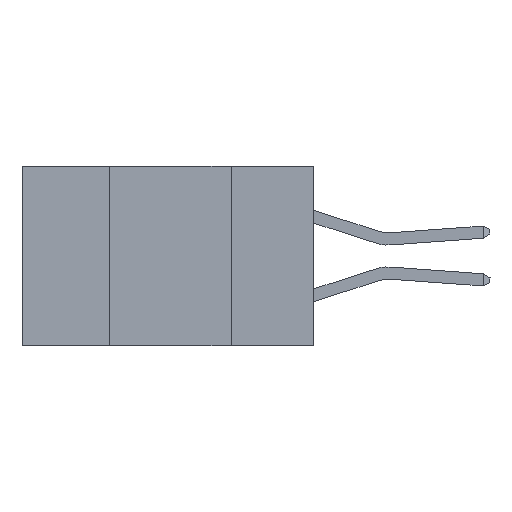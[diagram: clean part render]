
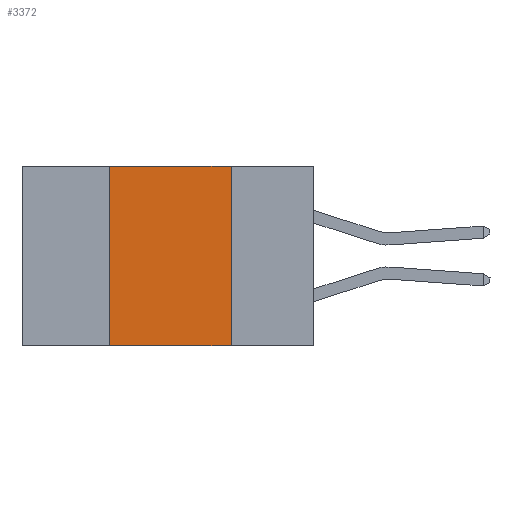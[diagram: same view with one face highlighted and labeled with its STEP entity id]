
A CAD part, left-side view. The second image highlights one B-rep face of the part: STEP entity #3372.
In plain terms, the highlighted planar face has unit normal (-1, 0, 0).
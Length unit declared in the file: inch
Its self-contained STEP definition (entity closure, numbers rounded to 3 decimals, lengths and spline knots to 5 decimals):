
#1549 = DIRECTION ( 'NONE',  ( 0., 0., -1. ) ) ;
#2661 = VECTOR ( 'NONE', #29546, 39.37008 ) ;
#3372 = ADVANCED_FACE ( 'NONE', ( #19261 ), #20694, .F. ) ;
#3659 = EDGE_CURVE ( 'NONE', #26814, #23594, #16336, .T. ) ;
#4311 = LINE ( 'NONE', #4772, #5348 ) ;
#4772 = CARTESIAN_POINT ( 'NONE',  ( 0., 0.6, 0. ) ) ;
#5348 = VECTOR ( 'NONE', #14231, 39.37008 ) ;
#6186 = VECTOR ( 'NONE', #18472, 39.37008 ) ;
#6596 = CARTESIAN_POINT ( 'NONE',  ( 0., 0.42, 0. ) ) ;
#7399 = CARTESIAN_POINT ( 'NONE',  ( 0., 0.17, 0. ) ) ;
#8484 = ORIENTED_EDGE ( 'NONE', *, *, #21941, .T. ) ;
#8750 = CARTESIAN_POINT ( 'NONE',  ( 0., 0.6, 0. ) ) ;
#10008 = EDGE_CURVE ( 'NONE', #28718, #22936, #15084, .T. ) ;
#10091 = CARTESIAN_POINT ( 'NONE',  ( 0., 0.42, -0.37 ) ) ;
#10804 = DIRECTION ( 'NONE',  ( 0., 0., 1. ) ) ;
#11940 = EDGE_CURVE ( 'NONE', #22936, #26814, #4311, .T. ) ;
#13475 = DIRECTION ( 'NONE',  ( 1., 0., 0. ) ) ;
#13518 = EDGE_LOOP ( 'NONE', ( #14694, #15448, #28871, #8484 ) ) ;
#14231 = DIRECTION ( 'NONE',  ( 0., -1., 0. ) ) ;
#14600 = AXIS2_PLACEMENT_3D ( 'NONE', #8750, #13475, #1549 ) ;
#14694 = ORIENTED_EDGE ( 'NONE', *, *, #3659, .F. ) ;
#15084 = LINE ( 'NONE', #6596, #22880 ) ;
#15448 = ORIENTED_EDGE ( 'NONE', *, *, #11940, .F. ) ;
#16336 = LINE ( 'NONE', #7399, #2661 ) ;
#16903 = CARTESIAN_POINT ( 'NONE',  ( 0., 0.42, 0. ) ) ;
#18472 = DIRECTION ( 'NONE',  ( 0., -1., 0. ) ) ;
#19261 = FACE_OUTER_BOUND ( 'NONE', #13518, .T. ) ;
#19815 = CARTESIAN_POINT ( 'NONE',  ( 0., 0.17, 0. ) ) ;
#20694 = PLANE ( 'NONE',  #14600 ) ;
#21941 = EDGE_CURVE ( 'NONE', #28718, #23594, #26781, .T. ) ;
#22880 = VECTOR ( 'NONE', #10804, 39.37008 ) ;
#22936 = VERTEX_POINT ( 'NONE', #16903 ) ;
#23412 = CARTESIAN_POINT ( 'NONE',  ( 0., 0.6, -0.37 ) ) ;
#23594 = VERTEX_POINT ( 'NONE', #28920 ) ;
#26781 = LINE ( 'NONE', #23412, #6186 ) ;
#26814 = VERTEX_POINT ( 'NONE', #19815 ) ;
#28718 = VERTEX_POINT ( 'NONE', #10091 ) ;
#28871 = ORIENTED_EDGE ( 'NONE', *, *, #10008, .F. ) ;
#28920 = CARTESIAN_POINT ( 'NONE',  ( 0., 0.17, -0.37 ) ) ;
#29546 = DIRECTION ( 'NONE',  ( 0., 0., -1. ) ) ;
